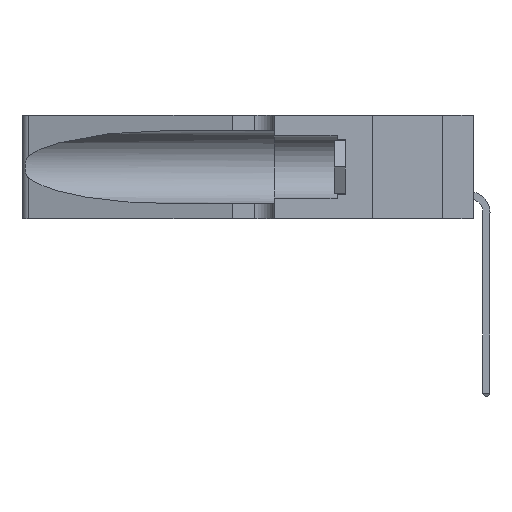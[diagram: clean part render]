
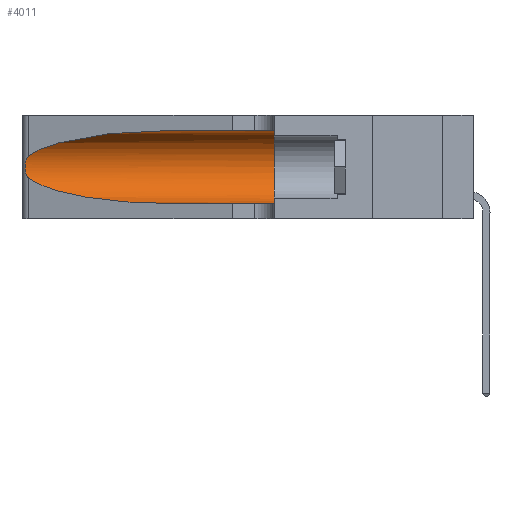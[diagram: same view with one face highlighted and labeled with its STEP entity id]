
A CAD part, left-side view. The second image highlights one B-rep face of the part: STEP entity #4011.
In plain terms, the highlighted cylindrical face has radius 3.308 mm (diameter 6.617 mm), a partial arc.
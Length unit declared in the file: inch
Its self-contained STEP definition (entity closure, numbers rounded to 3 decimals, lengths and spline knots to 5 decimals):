
#1863 = DIRECTION ( 'NONE',  ( 0., -1., 0. ) ) ;
#2205 = CARTESIAN_POINT ( 'NONE',  ( 0.18966, 0.96281, 0.31525 ) ) ;
#2604 = CARTESIAN_POINT ( 'NONE',  ( 0.25487, 1.22718, 0.22369 ) ) ;
#2643 = EDGE_LOOP ( 'NONE', ( #10458, #13603, #13564, #24281, #36578, #13932 ) ) ;
#3388 = DIRECTION ( 'NONE',  ( 0., -1., 0. ) ) ;
#4011 = ADVANCED_FACE ( 'NONE', ( #30741 ), #6332, .F. ) ;
#4202 = CARTESIAN_POINT ( 'NONE',  ( 0.1305, 0.35, 0.185 ) ) ;
#4256 = CARTESIAN_POINT ( 'NONE',  ( 0.1305, 1.61858, 0.31525 ) ) ;
#4377 = CARTESIAN_POINT ( 'NONE',  ( 0.25487, 1.22718, 0.22369 ) ) ;
#4393 = VERTEX_POINT ( 'NONE', #21209 ) ;
#4558 = LINE ( 'NONE', #4256, #33698 ) ;
#5881 =( BOUNDED_CURVE ( )  B_SPLINE_CURVE ( 3, ( #17531, #2205, #11679, #2604 ),
 .UNSPECIFIED., .F., .F. ) 
 B_SPLINE_CURVE_WITH_KNOTS ( ( 4, 4 ),
 ( 1.5708, 2.84003 ),
 .UNSPECIFIED. ) 
 CURVE ( )  GEOMETRIC_REPRESENTATION_ITEM ( )  RATIONAL_B_SPLINE_CURVE ( ( 1., 0.87, 0.87, 1. ) ) 
 REPRESENTATION_ITEM ( '' )  );
#6332 = CYLINDRICAL_SURFACE ( 'NONE', #37113, 0.13025 ) ;
#8076 = CARTESIAN_POINT ( 'NONE',  ( 0.26017, 1.23833, 0.17102 ) ) ;
#8107 = CARTESIAN_POINT ( 'NONE',  ( 0.18966, 0.96281, 0.05475 ) ) ;
#8384 = CARTESIAN_POINT ( 'NONE',  ( 0.25487, 1.22718, 0.14631 ) ) ;
#10011 = B_SPLINE_CURVE_WITH_KNOTS ( 'NONE', 3,
 ( #26754, #23258, #23531, #32770, #14077, #17147, #26345, #14475, #8076, #29417, #32504, #35850, #17543, #38902 ),
 .UNSPECIFIED., .F., .F.,
 ( 4, 2, 2, 2, 2, 2, 4 ),
 ( 0., 0.00027, 0.00053, 0.00107, 0.0016, 0.00187, 0.00214 ),
 .UNSPECIFIED. ) ;
#10458 = ORIENTED_EDGE ( 'NONE', *, *, #18290, .T. ) ;
#10515 = EDGE_CURVE ( 'NONE', #27198, #16792, #14651, .T. ) ;
#11473 = EDGE_CURVE ( 'NONE', #21757, #4393, #4558, .T. ) ;
#11679 = CARTESIAN_POINT ( 'NONE',  ( 0.2373, 1.15595, 0.28018 ) ) ;
#12229 = CARTESIAN_POINT ( 'NONE',  ( 0.25487, 1.22718, 0.14631 ) ) ;
#12535 = VERTEX_POINT ( 'NONE', #4377 ) ;
#13564 = ORIENTED_EDGE ( 'NONE', *, *, #37987, .T. ) ;
#13603 = ORIENTED_EDGE ( 'NONE', *, *, #35190, .T. ) ;
#13932 = ORIENTED_EDGE ( 'NONE', *, *, #11473, .F. ) ;
#14077 = CARTESIAN_POINT ( 'NONE',  ( 0.25854, 1.2359, 0.20912 ) ) ;
#14336 = CARTESIAN_POINT ( 'NONE',  ( 0.1305, 1.61858, 0.05475 ) ) ;
#14475 = CARTESIAN_POINT ( 'NONE',  ( 0.26075, 1.23896, 0.178 ) ) ;
#14651 = LINE ( 'NONE', #14336, #18469 ) ;
#16792 = VERTEX_POINT ( 'NONE', #27977 ) ;
#17147 = CARTESIAN_POINT ( 'NONE',  ( 0.26018, 1.23835, 0.19895 ) ) ;
#17531 = CARTESIAN_POINT ( 'NONE',  ( 0.1305, 0.72297, 0.31525 ) ) ;
#17543 = CARTESIAN_POINT ( 'NONE',  ( 0.25555, 1.22993, 0.14849 ) ) ;
#18290 = EDGE_CURVE ( 'NONE', #21757, #12535, #5881, .T. ) ;
#18469 = VECTOR ( 'NONE', #3388, 39.37008 ) ;
#20452 = EDGE_CURVE ( 'NONE', #4393, #16792, #24488, .T. ) ;
#20533 = DIRECTION ( 'NONE',  ( 0., -1., 0. ) ) ;
#20722 = CARTESIAN_POINT ( 'NONE',  ( 0.1305, 0.72297, 0.31525 ) ) ;
#21209 = CARTESIAN_POINT ( 'NONE',  ( 0.1305, 0.35, 0.31525 ) ) ;
#21757 = VERTEX_POINT ( 'NONE', #20722 ) ;
#23258 = CARTESIAN_POINT ( 'NONE',  ( 0.25555, 1.22994, 0.2215 ) ) ;
#23531 = CARTESIAN_POINT ( 'NONE',  ( 0.25639, 1.23184, 0.21858 ) ) ;
#24281 = ORIENTED_EDGE ( 'NONE', *, *, #10515, .T. ) ;
#24488 = CIRCLE ( 'NONE', #27908, 0.13025 ) ;
#26251 = CARTESIAN_POINT ( 'NONE',  ( 0.1305, 0.72297, 0.05475 ) ) ;
#26345 = CARTESIAN_POINT ( 'NONE',  ( 0.26075, 1.23896, 0.19203 ) ) ;
#26754 = CARTESIAN_POINT ( 'NONE',  ( 0.25487, 1.22718, 0.22369 ) ) ;
#27198 = VERTEX_POINT ( 'NONE', #39215 ) ;
#27908 = AXIS2_PLACEMENT_3D ( 'NONE', #4202, #31515, #39027 ) ;
#27977 = CARTESIAN_POINT ( 'NONE',  ( 0.1305, 0.35, 0.05475 ) ) ;
#29417 = CARTESIAN_POINT ( 'NONE',  ( 0.25856, 1.23593, 0.16098 ) ) ;
#30741 = FACE_OUTER_BOUND ( 'NONE', #2643, .T. ) ;
#31515 = DIRECTION ( 'NONE',  ( 0., 1., 0. ) ) ;
#32504 = CARTESIAN_POINT ( 'NONE',  ( 0.25789, 1.23486, 0.15765 ) ) ;
#32770 = CARTESIAN_POINT ( 'NONE',  ( 0.25787, 1.23484, 0.2124 ) ) ;
#32855 = DIRECTION ( 'NONE',  ( 0., 0., -1. ) ) ;
#32986 = CARTESIAN_POINT ( 'NONE',  ( 0.1305, 1.61858, 0.185 ) ) ;
#33407 = VERTEX_POINT ( 'NONE', #12229 ) ;
#33698 = VECTOR ( 'NONE', #1863, 39.37008 ) ;
#34251 =( BOUNDED_CURVE ( )  B_SPLINE_CURVE ( 3, ( #8384, #35357, #8107, #26251 ),
 .UNSPECIFIED., .F., .T. ) 
 B_SPLINE_CURVE_WITH_KNOTS ( ( 4, 4 ),
 ( 3.44316, 4.71239 ),
 .UNSPECIFIED. ) 
 CURVE ( )  GEOMETRIC_REPRESENTATION_ITEM ( )  RATIONAL_B_SPLINE_CURVE ( ( 1., 0.87, 0.87, 1. ) ) 
 REPRESENTATION_ITEM ( '' )  );
#35190 = EDGE_CURVE ( 'NONE', #12535, #33407, #10011, .T. ) ;
#35357 = CARTESIAN_POINT ( 'NONE',  ( 0.2373, 1.15595, 0.08982 ) ) ;
#35850 = CARTESIAN_POINT ( 'NONE',  ( 0.25639, 1.23186, 0.15144 ) ) ;
#36578 = ORIENTED_EDGE ( 'NONE', *, *, #20452, .F. ) ;
#37113 = AXIS2_PLACEMENT_3D ( 'NONE', #32986, #20533, #32855 ) ;
#37987 = EDGE_CURVE ( 'NONE', #33407, #27198, #34251, .T. ) ;
#38902 = CARTESIAN_POINT ( 'NONE',  ( 0.25487, 1.22718, 0.14631 ) ) ;
#39027 = DIRECTION ( 'NONE',  ( 0., 0., 1. ) ) ;
#39215 = CARTESIAN_POINT ( 'NONE',  ( 0.1305, 0.72297, 0.05475 ) ) ;
